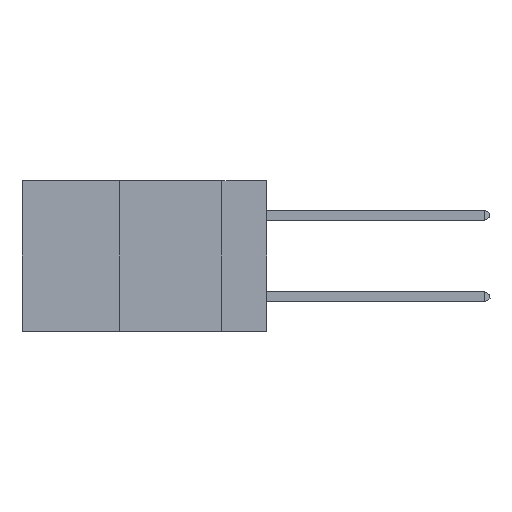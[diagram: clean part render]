
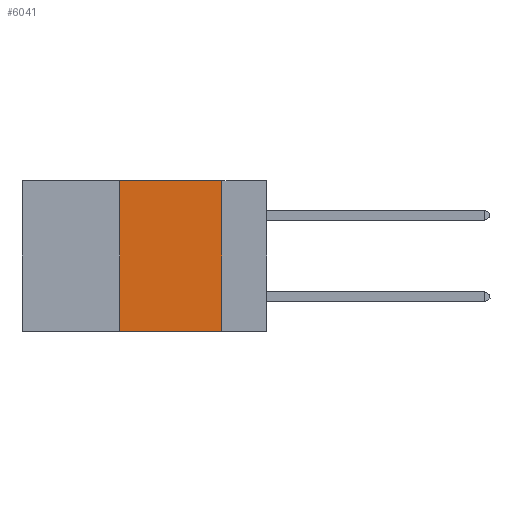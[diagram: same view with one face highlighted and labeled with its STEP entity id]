
A CAD part, left-side view. The second image highlights one B-rep face of the part: STEP entity #6041.
In plain terms, the highlighted planar face has unit normal (-1, 0, 0).
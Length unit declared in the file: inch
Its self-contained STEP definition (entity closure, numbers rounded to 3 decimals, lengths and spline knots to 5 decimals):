
#487 = LINE ( 'NONE', #13492, #11047 ) ;
#1684 = VECTOR ( 'NONE', #8881, 39.37008 ) ;
#1878 = CARTESIAN_POINT ( 'NONE',  ( 0., 0.11, 0. ) ) ;
#2804 = CARTESIAN_POINT ( 'NONE',  ( 0., 0.11, 0. ) ) ;
#3344 = CARTESIAN_POINT ( 'NONE',  ( 0., 0.36, -0.37 ) ) ;
#3485 = CARTESIAN_POINT ( 'NONE',  ( 0., 0.6, 0. ) ) ;
#4560 = VERTEX_POINT ( 'NONE', #11769 ) ;
#5108 = VECTOR ( 'NONE', #15721, 39.37008 ) ;
#5192 = VERTEX_POINT ( 'NONE', #3344 ) ;
#6041 = ADVANCED_FACE ( 'NONE', ( #9373 ), #6712, .F. ) ;
#6712 = PLANE ( 'NONE',  #9279 ) ;
#7520 = EDGE_CURVE ( 'NONE', #4560, #19454, #11107, .T. ) ;
#8069 = ORIENTED_EDGE ( 'NONE', *, *, #7520, .F. ) ;
#8491 = DIRECTION ( 'NONE',  ( 0., 0., -1. ) ) ;
#8597 = ORIENTED_EDGE ( 'NONE', *, *, #11109, .F. ) ;
#8881 = DIRECTION ( 'NONE',  ( 0., -1., 0. ) ) ;
#9279 = AXIS2_PLACEMENT_3D ( 'NONE', #13463, #18307, #8491 ) ;
#9373 = FACE_OUTER_BOUND ( 'NONE', #13405, .T. ) ;
#9973 = DIRECTION ( 'NONE',  ( 0., 0., -1. ) ) ;
#10999 = EDGE_CURVE ( 'NONE', #19454, #15041, #20178, .T. ) ;
#11047 = VECTOR ( 'NONE', #16573, 39.37008 ) ;
#11107 = LINE ( 'NONE', #3485, #1684 ) ;
#11109 = EDGE_CURVE ( 'NONE', #5192, #4560, #487, .T. ) ;
#11769 = CARTESIAN_POINT ( 'NONE',  ( 0., 0.36, 0. ) ) ;
#12096 = VECTOR ( 'NONE', #9973, 39.37008 ) ;
#13405 = EDGE_LOOP ( 'NONE', ( #20650, #8069, #8597, #21653 ) ) ;
#13463 = CARTESIAN_POINT ( 'NONE',  ( 0., 0.6, 0. ) ) ;
#13492 = CARTESIAN_POINT ( 'NONE',  ( 0., 0.36, 0. ) ) ;
#13678 = LINE ( 'NONE', #14199, #5108 ) ;
#14199 = CARTESIAN_POINT ( 'NONE',  ( 0., 0.6, -0.37 ) ) ;
#15041 = VERTEX_POINT ( 'NONE', #19434 ) ;
#15455 = EDGE_CURVE ( 'NONE', #5192, #15041, #13678, .T. ) ;
#15721 = DIRECTION ( 'NONE',  ( 0., -1., 0. ) ) ;
#16573 = DIRECTION ( 'NONE',  ( 0., 0., 1. ) ) ;
#18307 = DIRECTION ( 'NONE',  ( 1., 0., 0. ) ) ;
#19434 = CARTESIAN_POINT ( 'NONE',  ( 0., 0.11, -0.37 ) ) ;
#19454 = VERTEX_POINT ( 'NONE', #1878 ) ;
#20178 = LINE ( 'NONE', #2804, #12096 ) ;
#20650 = ORIENTED_EDGE ( 'NONE', *, *, #10999, .F. ) ;
#21653 = ORIENTED_EDGE ( 'NONE', *, *, #15455, .T. ) ;
